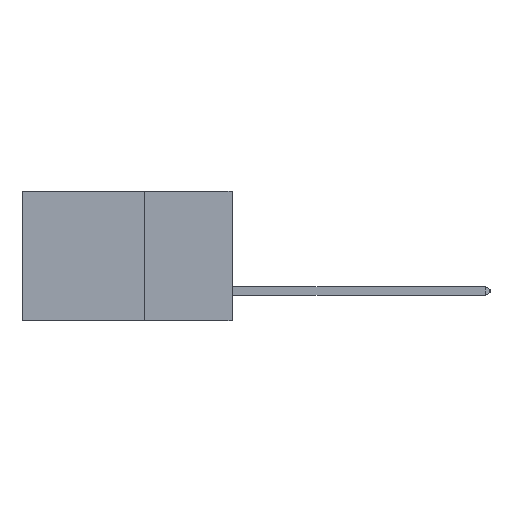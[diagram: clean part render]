
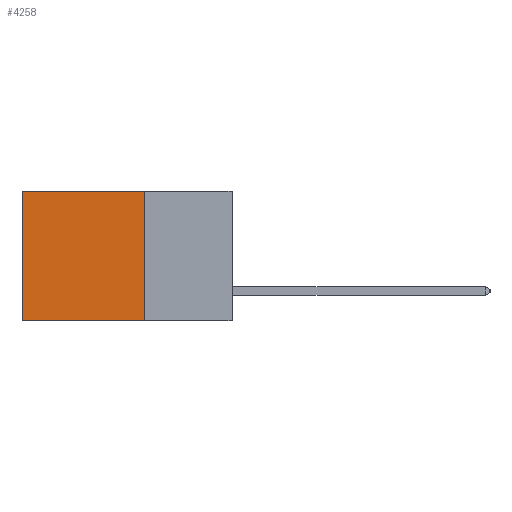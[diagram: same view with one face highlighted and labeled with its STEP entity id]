
A CAD part, left-side view. The second image highlights one B-rep face of the part: STEP entity #4258.
In plain terms, the highlighted planar face has unit normal (-1, 0, 0).
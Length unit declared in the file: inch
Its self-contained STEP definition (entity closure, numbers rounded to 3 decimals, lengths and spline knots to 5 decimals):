
#51 = DIRECTION ( 'NONE',  ( 1., 0., 0. ) ) ;
#88 = AXIS2_PLACEMENT_3D ( 'NONE', #15269, #51, #17818 ) ;
#327 = CARTESIAN_POINT ( 'NONE',  ( 0.2875, 0.25, 0. ) ) ;
#619 = ORIENTED_EDGE ( 'NONE', *, *, #12240, .F. ) ;
#2819 = EDGE_CURVE ( 'NONE', #21482, #20020, #19875, .T. ) ;
#3118 = CARTESIAN_POINT ( 'NONE',  ( 0.2875, 0.25, 0. ) ) ;
#4258 = ADVANCED_FACE ( 'NONE', ( #16596 ), #20293, .F. ) ;
#5012 = EDGE_CURVE ( 'NONE', #21482, #12458, #31571, .T. ) ;
#5646 = DIRECTION ( 'NONE',  ( 0., 0., -1. ) ) ;
#7293 = CARTESIAN_POINT ( 'NONE',  ( 0.2875, 0.6, 0. ) ) ;
#7590 = DIRECTION ( 'NONE',  ( 0., 1., 0. ) ) ;
#9308 = DIRECTION ( 'NONE',  ( 0., 1., 0. ) ) ;
#9830 = DIRECTION ( 'NONE',  ( 0., 0., -1. ) ) ;
#11348 = VECTOR ( 'NONE', #5646, 39.37008 ) ;
#11825 = VECTOR ( 'NONE', #7590, 39.37008 ) ;
#12240 = EDGE_CURVE ( 'NONE', #12458, #12792, #24516, .T. ) ;
#12458 = VERTEX_POINT ( 'NONE', #16262 ) ;
#12792 = VERTEX_POINT ( 'NONE', #15006 ) ;
#15006 = CARTESIAN_POINT ( 'NONE',  ( 0.2875, 0.6, -0.37 ) ) ;
#15269 = CARTESIAN_POINT ( 'NONE',  ( 0.2875, 0.25, 0. ) ) ;
#15882 = EDGE_LOOP ( 'NONE', ( #22978, #619, #23297, #19604 ) ) ;
#16262 = CARTESIAN_POINT ( 'NONE',  ( 0.2875, 0.25, -0.37 ) ) ;
#16596 = FACE_OUTER_BOUND ( 'NONE', #15882, .T. ) ;
#17818 = DIRECTION ( 'NONE',  ( 0., 0., -1. ) ) ;
#19604 = ORIENTED_EDGE ( 'NONE', *, *, #2819, .T. ) ;
#19875 = LINE ( 'NONE', #24520, #32519 ) ;
#20020 = VERTEX_POINT ( 'NONE', #29773 ) ;
#20293 = PLANE ( 'NONE',  #88 ) ;
#21482 = VERTEX_POINT ( 'NONE', #327 ) ;
#22827 = CARTESIAN_POINT ( 'NONE',  ( 0.2875, 0.25, -0.37 ) ) ;
#22978 = ORIENTED_EDGE ( 'NONE', *, *, #26047, .T. ) ;
#23297 = ORIENTED_EDGE ( 'NONE', *, *, #5012, .F. ) ;
#24516 = LINE ( 'NONE', #22827, #11825 ) ;
#24520 = CARTESIAN_POINT ( 'NONE',  ( 0.2875, 0.25, 0. ) ) ;
#26047 = EDGE_CURVE ( 'NONE', #20020, #12792, #30663, .T. ) ;
#29773 = CARTESIAN_POINT ( 'NONE',  ( 0.2875, 0.6, 0. ) ) ;
#29852 = VECTOR ( 'NONE', #9830, 39.37008 ) ;
#30663 = LINE ( 'NONE', #7293, #29852 ) ;
#31571 = LINE ( 'NONE', #3118, #11348 ) ;
#32519 = VECTOR ( 'NONE', #9308, 39.37008 ) ;
